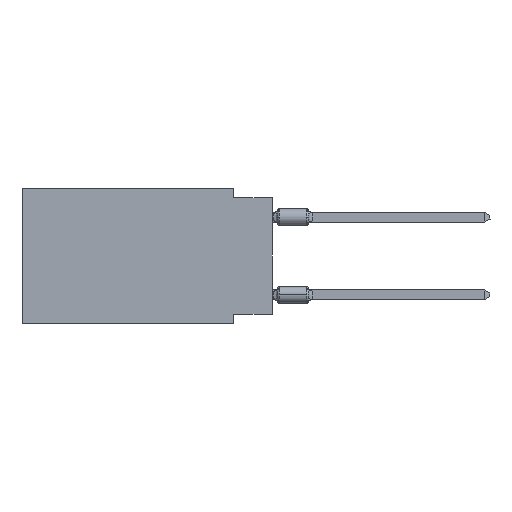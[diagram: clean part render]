
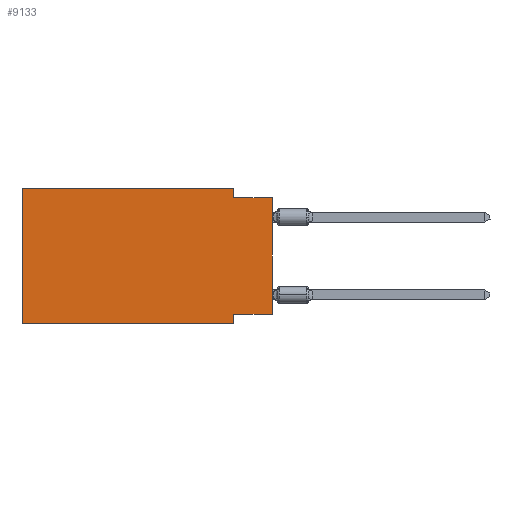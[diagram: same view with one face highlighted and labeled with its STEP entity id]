
A CAD part, left-side view. The second image highlights one B-rep face of the part: STEP entity #9133.
In plain terms, the highlighted planar face has unit normal (-1, 0, 0).
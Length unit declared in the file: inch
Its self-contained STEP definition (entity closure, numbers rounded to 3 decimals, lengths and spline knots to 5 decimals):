
#1631 = FACE_OUTER_BOUND ( 'NONE', #33062, .T. ) ;
#2947 = EDGE_CURVE ( 'NONE', #18156, #18974, #47337, .T. ) ;
#3113 = CARTESIAN_POINT ( 'NONE',  ( 0., 0.1, -0.325 ) ) ;
#4305 = CARTESIAN_POINT ( 'NONE',  ( 0., 0.645, -0.35 ) ) ;
#4400 = ORIENTED_EDGE ( 'NONE', *, *, #62552, .F. ) ;
#6060 = VERTEX_POINT ( 'NONE', #52633 ) ;
#6893 = EDGE_CURVE ( 'NONE', #30751, #18156, #30249, .T. ) ;
#7191 = ORIENTED_EDGE ( 'NONE', *, *, #42217, .F. ) ;
#7241 = DIRECTION ( 'NONE',  ( 0., 0., 1. ) ) ;
#7446 = DIRECTION ( 'NONE',  ( 1., 0., 0. ) ) ;
#7614 = LINE ( 'NONE', #57586, #42372 ) ;
#7810 = CARTESIAN_POINT ( 'NONE',  ( 0., 0.645, 0. ) ) ;
#8031 = ORIENTED_EDGE ( 'NONE', *, *, #14179, .T. ) ;
#9133 = ADVANCED_FACE ( 'NONE', ( #1631 ), #24206, .F. ) ;
#9152 = VECTOR ( 'NONE', #11668, 39.37008 ) ;
#10942 = ORIENTED_EDGE ( 'NONE', *, *, #14332, .T. ) ;
#11668 = DIRECTION ( 'NONE',  ( 0., 1., 0. ) ) ;
#11837 = LINE ( 'NONE', #57406, #20608 ) ;
#12544 = DIRECTION ( 'NONE',  ( 0., 0., 1. ) ) ;
#13192 = ORIENTED_EDGE ( 'NONE', *, *, #2947, .F. ) ;
#14179 = EDGE_CURVE ( 'NONE', #40894, #18974, #7614, .T. ) ;
#14332 = EDGE_CURVE ( 'NONE', #6060, #60173, #70663, .T. ) ;
#17705 = CARTESIAN_POINT ( 'NONE',  ( 0., 0.1, 0. ) ) ;
#17709 = VERTEX_POINT ( 'NONE', #26783 ) ;
#18156 = VERTEX_POINT ( 'NONE', #28073 ) ;
#18974 = VERTEX_POINT ( 'NONE', #62860 ) ;
#20314 = VECTOR ( 'NONE', #54262, 39.37008 ) ;
#20608 = VECTOR ( 'NONE', #12544, 39.37008 ) ;
#21370 = DIRECTION ( 'NONE',  ( 0., -1., 0. ) ) ;
#21724 = CARTESIAN_POINT ( 'NONE',  ( 0., 0.645, 0. ) ) ;
#21851 = EDGE_CURVE ( 'NONE', #40955, #60173, #47248, .T. ) ;
#24206 = PLANE ( 'NONE',  #25783 ) ;
#25783 = AXIS2_PLACEMENT_3D ( 'NONE', #7810, #7446, #68698 ) ;
#26405 = ORIENTED_EDGE ( 'NONE', *, *, #21851, .F. ) ;
#26783 = CARTESIAN_POINT ( 'NONE',  ( 0., 0.645, 0. ) ) ;
#26809 = LINE ( 'NONE', #21724, #42675 ) ;
#27953 = DIRECTION ( 'NONE',  ( 0., -1., 0. ) ) ;
#28073 = CARTESIAN_POINT ( 'NONE',  ( 0., 0.1, -0.025 ) ) ;
#28080 = VECTOR ( 'NONE', #52505, 39.37008 ) ;
#28113 = ORIENTED_EDGE ( 'NONE', *, *, #6893, .F. ) ;
#28242 = CARTESIAN_POINT ( 'NONE',  ( 0., 0.1, -0.35 ) ) ;
#30249 = LINE ( 'NONE', #56901, #28080 ) ;
#30751 = VERTEX_POINT ( 'NONE', #17705 ) ;
#33062 = EDGE_LOOP ( 'NONE', ( #8031, #13192, #28113, #7191, #64720, #10942, #26405, #4400 ) ) ;
#37826 = CARTESIAN_POINT ( 'NONE',  ( 0., 0., -0.025 ) ) ;
#38656 = LINE ( 'NONE', #55449, #9152 ) ;
#40894 = VERTEX_POINT ( 'NONE', #62571 ) ;
#40955 = VERTEX_POINT ( 'NONE', #3113 ) ;
#42217 = EDGE_CURVE ( 'NONE', #17709, #30751, #26809, .T. ) ;
#42372 = VECTOR ( 'NONE', #7241, 39.37008 ) ;
#42675 = VECTOR ( 'NONE', #21370, 39.37008 ) ;
#43635 = VECTOR ( 'NONE', #64034, 39.37008 ) ;
#47248 = LINE ( 'NONE', #47962, #43635 ) ;
#47337 = LINE ( 'NONE', #37826, #60482 ) ;
#47962 = CARTESIAN_POINT ( 'NONE',  ( 0., 0.1, -0.35 ) ) ;
#52505 = DIRECTION ( 'NONE',  ( 0., 0., -1. ) ) ;
#52633 = CARTESIAN_POINT ( 'NONE',  ( 0., 0.645, -0.35 ) ) ;
#54262 = DIRECTION ( 'NONE',  ( 0., -1., 0. ) ) ;
#55449 = CARTESIAN_POINT ( 'NONE',  ( 0., 0., -0.325 ) ) ;
#56901 = CARTESIAN_POINT ( 'NONE',  ( 0., 0.1, 0. ) ) ;
#57406 = CARTESIAN_POINT ( 'NONE',  ( 0., 0.645, 0. ) ) ;
#57586 = CARTESIAN_POINT ( 'NONE',  ( 0., 0., 0. ) ) ;
#60161 = EDGE_CURVE ( 'NONE', #6060, #17709, #11837, .T. ) ;
#60173 = VERTEX_POINT ( 'NONE', #28242 ) ;
#60482 = VECTOR ( 'NONE', #27953, 39.37008 ) ;
#62552 = EDGE_CURVE ( 'NONE', #40894, #40955, #38656, .T. ) ;
#62571 = CARTESIAN_POINT ( 'NONE',  ( 0., 0., -0.325 ) ) ;
#62860 = CARTESIAN_POINT ( 'NONE',  ( 0., 0., -0.025 ) ) ;
#64034 = DIRECTION ( 'NONE',  ( 0., 0., -1. ) ) ;
#64720 = ORIENTED_EDGE ( 'NONE', *, *, #60161, .F. ) ;
#68698 = DIRECTION ( 'NONE',  ( 0., 0., -1. ) ) ;
#70663 = LINE ( 'NONE', #4305, #20314 ) ;
